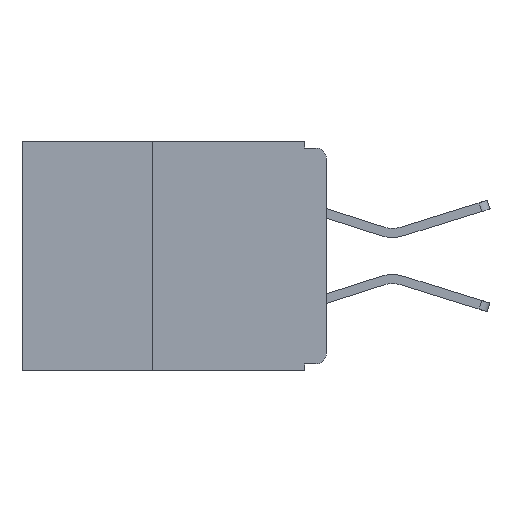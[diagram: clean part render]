
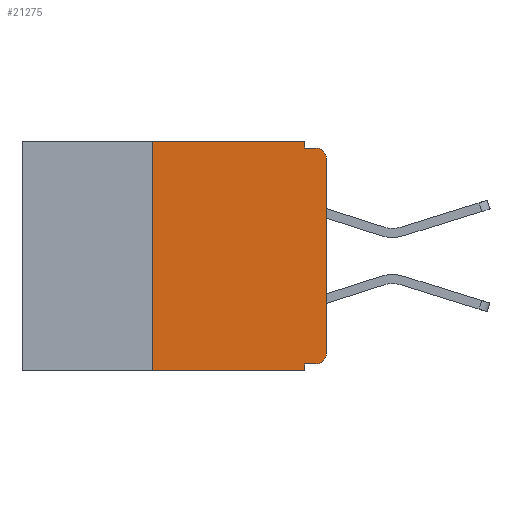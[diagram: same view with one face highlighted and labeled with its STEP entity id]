
A CAD part, left-side view. The second image highlights one B-rep face of the part: STEP entity #21275.
In plain terms, the highlighted planar face has unit normal (-1, 0, 0).
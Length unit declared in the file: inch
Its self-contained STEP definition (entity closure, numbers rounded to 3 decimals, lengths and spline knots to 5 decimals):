
#166 = ORIENTED_EDGE ( 'NONE', *, *, #24990, .T. ) ;
#1070 = LINE ( 'NONE', #17436, #6933 ) ;
#1648 = DIRECTION ( 'NONE',  ( 0., 0., -1. ) ) ;
#1822 = ORIENTED_EDGE ( 'NONE', *, *, #14013, .F. ) ;
#1956 = VERTEX_POINT ( 'NONE', #14301 ) ;
#2156 = VERTEX_POINT ( 'NONE', #25103 ) ;
#2846 = CARTESIAN_POINT ( 'NONE',  ( 0., 0., -0.32 ) ) ;
#3310 = VERTEX_POINT ( 'NONE', #4325 ) ;
#3363 = ORIENTED_EDGE ( 'NONE', *, *, #9578, .F. ) ;
#3558 = LINE ( 'NONE', #8868, #19138 ) ;
#3692 = CARTESIAN_POINT ( 'NONE',  ( 0., 0.015, -0.025 ) ) ;
#3704 = VECTOR ( 'NONE', #20136, 39.37008 ) ;
#3865 = AXIS2_PLACEMENT_3D ( 'NONE', #19561, #6953, #21648 ) ;
#4282 = VERTEX_POINT ( 'NONE', #12413 ) ;
#4325 = CARTESIAN_POINT ( 'NONE',  ( 0., 0.015, -0.01 ) ) ;
#4421 = AXIS2_PLACEMENT_3D ( 'NONE', #3692, #18516, #5924 ) ;
#5543 = CARTESIAN_POINT ( 'NONE',  ( 0., 0.031, 0. ) ) ;
#5556 = EDGE_CURVE ( 'NONE', #6323, #14702, #3558, .T. ) ;
#5805 = VECTOR ( 'NONE', #12421, 39.37008 ) ;
#5924 = DIRECTION ( 'NONE',  ( 0., 0., -1. ) ) ;
#6323 = VERTEX_POINT ( 'NONE', #5543 ) ;
#6909 = VECTOR ( 'NONE', #10720, 39.37008 ) ;
#6933 = VECTOR ( 'NONE', #11106, 39.37008 ) ;
#6953 = DIRECTION ( 'NONE',  ( -1., 0., 0. ) ) ;
#7141 = DIRECTION ( 'NONE',  ( 0., 1., 0. ) ) ;
#7330 = DIRECTION ( 'NONE',  ( 0., 0., -1. ) ) ;
#7558 = CIRCLE ( 'NONE', #3865, 0.015 ) ;
#8868 = CARTESIAN_POINT ( 'NONE',  ( 0., 0.031, 0. ) ) ;
#8895 = ORIENTED_EDGE ( 'NONE', *, *, #15222, .T. ) ;
#8995 = CARTESIAN_POINT ( 'NONE',  ( 0., 0., -0.305 ) ) ;
#9442 = FACE_OUTER_BOUND ( 'NONE', #26158, .T. ) ;
#9443 = CARTESIAN_POINT ( 'NONE',  ( 0., 0.031, -0.33 ) ) ;
#9578 = EDGE_CURVE ( 'NONE', #4282, #1956, #22855, .T. ) ;
#10460 = VECTOR ( 'NONE', #7330, 39.37008 ) ;
#10720 = DIRECTION ( 'NONE',  ( 0., -1., 0. ) ) ;
#10819 = ORIENTED_EDGE ( 'NONE', *, *, #11519, .F. ) ;
#11002 = DIRECTION ( 'NONE',  ( 0., 0., -1. ) ) ;
#11106 = DIRECTION ( 'NONE',  ( 0., -1., 0. ) ) ;
#11129 = LINE ( 'NONE', #9443, #10460 ) ;
#11519 = EDGE_CURVE ( 'NONE', #14702, #3310, #1070, .T. ) ;
#12379 = VECTOR ( 'NONE', #7141, 39.37008 ) ;
#12392 = ORIENTED_EDGE ( 'NONE', *, *, #5556, .F. ) ;
#12413 = CARTESIAN_POINT ( 'NONE',  ( 0., 0.015, -0.32 ) ) ;
#12421 = DIRECTION ( 'NONE',  ( 0., 0., 1. ) ) ;
#12729 = CARTESIAN_POINT ( 'NONE',  ( 0., 0.437, -0.33 ) ) ;
#14013 = EDGE_CURVE ( 'NONE', #26618, #2156, #27320, .T. ) ;
#14301 = CARTESIAN_POINT ( 'NONE',  ( 0., 0.031, -0.32 ) ) ;
#14345 = CIRCLE ( 'NONE', #4421, 0.015 ) ;
#14506 = DIRECTION ( 'NONE',  ( 1., 0., 0. ) ) ;
#14653 = AXIS2_PLACEMENT_3D ( 'NONE', #22813, #14506, #1648 ) ;
#14702 = VERTEX_POINT ( 'NONE', #27178 ) ;
#15222 = EDGE_CURVE ( 'NONE', #25050, #3310, #14345, .T. ) ;
#15921 = CARTESIAN_POINT ( 'NONE',  ( 0., 0.031, -0.33 ) ) ;
#15982 = ORIENTED_EDGE ( 'NONE', *, *, #17316, .F. ) ;
#16278 = EDGE_CURVE ( 'NONE', #25864, #25050, #19949, .T. ) ;
#17316 = EDGE_CURVE ( 'NONE', #2156, #6323, #26949, .T. ) ;
#17436 = CARTESIAN_POINT ( 'NONE',  ( 0., 0., -0.01 ) ) ;
#18018 = CARTESIAN_POINT ( 'NONE',  ( 0., 0., 0. ) ) ;
#18516 = DIRECTION ( 'NONE',  ( -1., 0., 0. ) ) ;
#19138 = VECTOR ( 'NONE', #11002, 39.37008 ) ;
#19392 = ORIENTED_EDGE ( 'NONE', *, *, #19649, .T. ) ;
#19561 = CARTESIAN_POINT ( 'NONE',  ( 0., 0.015, -0.305 ) ) ;
#19649 = EDGE_CURVE ( 'NONE', #26618, #22740, #23644, .T. ) ;
#19949 = LINE ( 'NONE', #18018, #3704 ) ;
#20136 = DIRECTION ( 'NONE',  ( 0., 0., 1. ) ) ;
#20501 = CARTESIAN_POINT ( 'NONE',  ( 0., 0.437, 0. ) ) ;
#21035 = EDGE_CURVE ( 'NONE', #1956, #22740, #11129, .T. ) ;
#21275 = ADVANCED_FACE ( 'NONE', ( #9442 ), #26922, .F. ) ;
#21648 = DIRECTION ( 'NONE',  ( 0., 0., -1. ) ) ;
#21902 = CARTESIAN_POINT ( 'NONE',  ( 0., 0.25, -0.33 ) ) ;
#22581 = DIRECTION ( 'NONE',  ( 0., -1., 0. ) ) ;
#22740 = VERTEX_POINT ( 'NONE', #15921 ) ;
#22813 = CARTESIAN_POINT ( 'NONE',  ( 0., 0.437, 0. ) ) ;
#22855 = LINE ( 'NONE', #2846, #12379 ) ;
#23407 = ORIENTED_EDGE ( 'NONE', *, *, #16278, .T. ) ;
#23644 = LINE ( 'NONE', #12729, #6909 ) ;
#24938 = CARTESIAN_POINT ( 'NONE',  ( 0., 0.25, -0.33 ) ) ;
#24990 = EDGE_CURVE ( 'NONE', #4282, #25864, #7558, .T. ) ;
#25050 = VERTEX_POINT ( 'NONE', #25971 ) ;
#25103 = CARTESIAN_POINT ( 'NONE',  ( 0., 0.25, 0. ) ) ;
#25864 = VERTEX_POINT ( 'NONE', #8995 ) ;
#25971 = CARTESIAN_POINT ( 'NONE',  ( 0., 0., -0.025 ) ) ;
#26158 = EDGE_LOOP ( 'NONE', ( #23407, #8895, #10819, #12392, #15982, #1822, #19392, #26214, #3363, #166 ) ) ;
#26214 = ORIENTED_EDGE ( 'NONE', *, *, #21035, .F. ) ;
#26340 = VECTOR ( 'NONE', #22581, 39.37008 ) ;
#26618 = VERTEX_POINT ( 'NONE', #21902 ) ;
#26922 = PLANE ( 'NONE',  #14653 ) ;
#26949 = LINE ( 'NONE', #20501, #26340 ) ;
#27178 = CARTESIAN_POINT ( 'NONE',  ( 0., 0.031, -0.01 ) ) ;
#27320 = LINE ( 'NONE', #24938, #5805 ) ;
